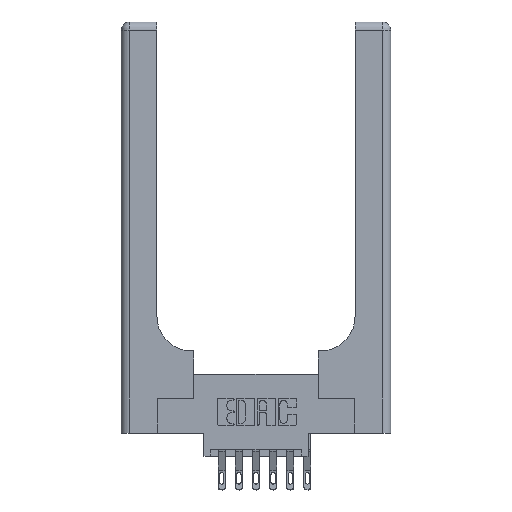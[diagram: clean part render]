
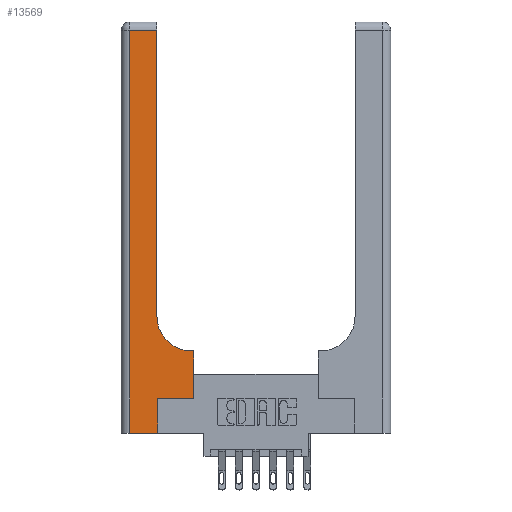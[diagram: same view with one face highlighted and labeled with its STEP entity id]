
A CAD part, top view. The second image highlights one B-rep face of the part: STEP entity #13569.
In plain terms, the highlighted planar face has unit normal (0, 0, 1).
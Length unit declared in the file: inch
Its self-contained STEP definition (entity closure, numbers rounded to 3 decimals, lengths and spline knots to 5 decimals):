
#8 = AXIS2_PLACEMENT_3D ( 'NONE', #514, #4835, #3612 ) ;
#164 = CARTESIAN_POINT ( 'NONE',  ( 0.26, 0.6, 0.37 ) ) ;
#227 = VECTOR ( 'NONE', #8159, 39.37008 ) ;
#239 = CARTESIAN_POINT ( 'NONE',  ( 0.26, 0.85, 0.37 ) ) ;
#422 = CARTESIAN_POINT ( 'NONE',  ( 0.265, 0.25, 0.37 ) ) ;
#514 = CARTESIAN_POINT ( 'NONE',  ( 0.51, 0.85, 0.37 ) ) ;
#1358 = EDGE_CURVE ( 'NONE', #9480, #7232, #2733, .T. ) ;
#1396 = DIRECTION ( 'NONE',  ( 0., 1., 0. ) ) ;
#1518 = ORIENTED_EDGE ( 'NONE', *, *, #12846, .T. ) ;
#1558 = ORIENTED_EDGE ( 'NONE', *, *, #10433, .T. ) ;
#1927 = EDGE_CURVE ( 'NONE', #5930, #9480, #6247, .T. ) ;
#2445 = LINE ( 'NONE', #164, #10129 ) ;
#2537 = ORIENTED_EDGE ( 'NONE', *, *, #10858, .T. ) ;
#2606 = VERTEX_POINT ( 'NONE', #5038 ) ;
#2679 = LINE ( 'NONE', #6259, #7978 ) ;
#2733 = LINE ( 'NONE', #11590, #227 ) ;
#2808 = CARTESIAN_POINT ( 'NONE',  ( 0.06, 0., 0.37 ) ) ;
#3612 = DIRECTION ( 'NONE',  ( 1., 0., 0. ) ) ;
#3621 = LINE ( 'NONE', #11311, #8699 ) ;
#4074 = CARTESIAN_POINT ( 'NONE',  ( 0.265, 0., 0.37 ) ) ;
#4299 = CARTESIAN_POINT ( 'NONE',  ( 0.265, 0.25, 0.37 ) ) ;
#4816 = DIRECTION ( 'NONE',  ( 1., 0., 0. ) ) ;
#4835 = DIRECTION ( 'NONE',  ( 0., 0., -1. ) ) ;
#4882 = VECTOR ( 'NONE', #14094, 39.37008 ) ;
#4993 = CARTESIAN_POINT ( 'NONE',  ( 0.51, 0.6, 0.37 ) ) ;
#5021 = LINE ( 'NONE', #4074, #4882 ) ;
#5033 = EDGE_CURVE ( 'NONE', #8871, #8685, #10404, .T. ) ;
#5038 = CARTESIAN_POINT ( 'NONE',  ( 0.06, 2.94, 0.37 ) ) ;
#5139 = ORIENTED_EDGE ( 'NONE', *, *, #10271, .T. ) ;
#5162 = VECTOR ( 'NONE', #14101, 39.37008 ) ;
#5686 = PLANE ( 'NONE',  #12059 ) ;
#5743 = CARTESIAN_POINT ( 'NONE',  ( 0., 3., 0.37 ) ) ;
#5776 = VERTEX_POINT ( 'NONE', #2808 ) ;
#5930 = VERTEX_POINT ( 'NONE', #4993 ) ;
#6053 = VECTOR ( 'NONE', #4816, 39.37008 ) ;
#6247 = CIRCLE ( 'NONE', #8, 0.25 ) ;
#6259 = CARTESIAN_POINT ( 'NONE',  ( 0.06, 3., 0.37 ) ) ;
#6713 = ORIENTED_EDGE ( 'NONE', *, *, #1358, .T. ) ;
#7087 = DIRECTION ( 'NONE',  ( 1., 0., 0. ) ) ;
#7144 = CARTESIAN_POINT ( 'NONE',  ( 0., 2.94, 0.37 ) ) ;
#7232 = VERTEX_POINT ( 'NONE', #7925 ) ;
#7446 = CARTESIAN_POINT ( 'NONE',  ( 0.528, 0.25, 0.37 ) ) ;
#7925 = CARTESIAN_POINT ( 'NONE',  ( 0.26, 2.94, 0.37 ) ) ;
#7978 = VECTOR ( 'NONE', #8391, 39.37008 ) ;
#8022 = DIRECTION ( 'NONE',  ( 0., 0., -1. ) ) ;
#8159 = DIRECTION ( 'NONE',  ( 0., 1., 0. ) ) ;
#8391 = DIRECTION ( 'NONE',  ( 0., -1., 0. ) ) ;
#8685 = VERTEX_POINT ( 'NONE', #7446 ) ;
#8699 = VECTOR ( 'NONE', #1396, 39.37008 ) ;
#8871 = VERTEX_POINT ( 'NONE', #4299 ) ;
#9271 = VECTOR ( 'NONE', #7087, 39.37008 ) ;
#9480 = VERTEX_POINT ( 'NONE', #239 ) ;
#9979 = VERTEX_POINT ( 'NONE', #11987 ) ;
#10023 = ORIENTED_EDGE ( 'NONE', *, *, #1927, .T. ) ;
#10129 = VECTOR ( 'NONE', #13621, 39.37008 ) ;
#10171 = FACE_OUTER_BOUND ( 'NONE', #10884, .T. ) ;
#10271 = EDGE_CURVE ( 'NONE', #2606, #5776, #2679, .T. ) ;
#10381 = ORIENTED_EDGE ( 'NONE', *, *, #11129, .T. ) ;
#10404 = LINE ( 'NONE', #422, #6053 ) ;
#10433 = EDGE_CURVE ( 'NONE', #8685, #13118, #3621, .T. ) ;
#10539 = LINE ( 'NONE', #11347, #9271 ) ;
#10641 = DIRECTION ( 'NONE',  ( -1., 0., 0. ) ) ;
#10858 = EDGE_CURVE ( 'NONE', #13118, #5930, #2445, .T. ) ;
#10884 = EDGE_LOOP ( 'NONE', ( #6713, #10381, #5139, #1518, #14385, #14247, #1558, #2537, #10023 ) ) ;
#11129 = EDGE_CURVE ( 'NONE', #7232, #2606, #14021, .T. ) ;
#11311 = CARTESIAN_POINT ( 'NONE',  ( 0.528, 0.25, 0.37 ) ) ;
#11347 = CARTESIAN_POINT ( 'NONE',  ( 0., 0., 0.37 ) ) ;
#11590 = CARTESIAN_POINT ( 'NONE',  ( 0.26, 3., 0.37 ) ) ;
#11987 = CARTESIAN_POINT ( 'NONE',  ( 0.265, 0., 0.37 ) ) ;
#12059 = AXIS2_PLACEMENT_3D ( 'NONE', #5743, #8022, #10641 ) ;
#12846 = EDGE_CURVE ( 'NONE', #5776, #9979, #10539, .T. ) ;
#13118 = VERTEX_POINT ( 'NONE', #14393 ) ;
#13243 = EDGE_CURVE ( 'NONE', #9979, #8871, #5021, .T. ) ;
#13569 = ADVANCED_FACE ( 'NONE', ( #10171 ), #5686, .F. ) ;
#13621 = DIRECTION ( 'NONE',  ( -1., 0., 0. ) ) ;
#14021 = LINE ( 'NONE', #7144, #5162 ) ;
#14094 = DIRECTION ( 'NONE',  ( 0., 1., 0. ) ) ;
#14101 = DIRECTION ( 'NONE',  ( -1., 0., 0. ) ) ;
#14247 = ORIENTED_EDGE ( 'NONE', *, *, #5033, .T. ) ;
#14385 = ORIENTED_EDGE ( 'NONE', *, *, #13243, .T. ) ;
#14393 = CARTESIAN_POINT ( 'NONE',  ( 0.528, 0.6, 0.37 ) ) ;
